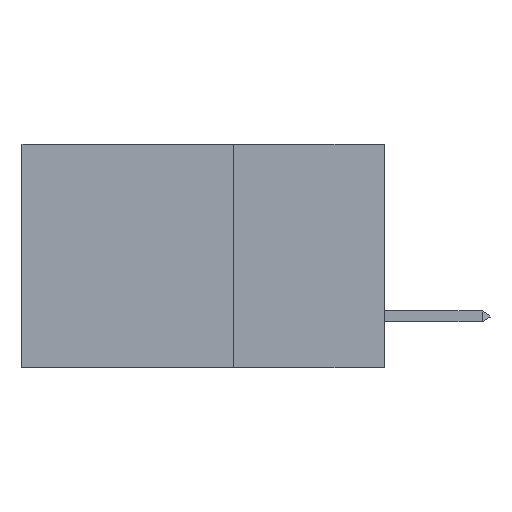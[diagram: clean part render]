
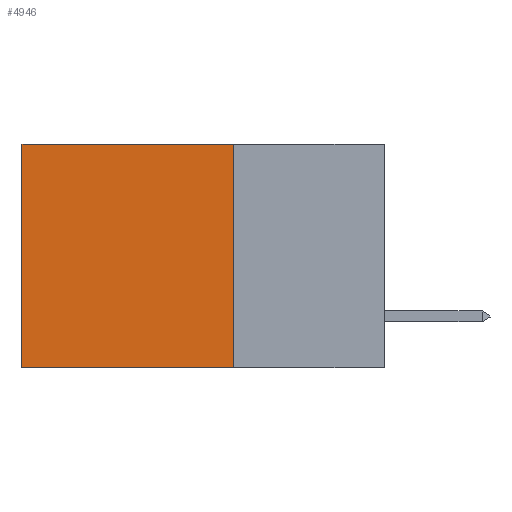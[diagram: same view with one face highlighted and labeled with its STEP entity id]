
A CAD part, left-side view. The second image highlights one B-rep face of the part: STEP entity #4946.
In plain terms, the highlighted planar face has unit normal (-1, 0, 0).
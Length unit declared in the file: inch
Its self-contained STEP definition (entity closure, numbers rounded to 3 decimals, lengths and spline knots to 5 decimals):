
#54 = VECTOR ( 'NONE', #7516, 39.37008 ) ;
#620 = VECTOR ( 'NONE', #25368, 39.37008 ) ;
#838 = EDGE_CURVE ( 'NONE', #45967, #17429, #23193, .T. ) ;
#1582 = CARTESIAN_POINT ( 'NONE',  ( 0.2875, 0.25, -0.37 ) ) ;
#3534 = LINE ( 'NONE', #39984, #35358 ) ;
#4235 = ORIENTED_EDGE ( 'NONE', *, *, #838, .T. ) ;
#4244 = ORIENTED_EDGE ( 'NONE', *, *, #40751, .F. ) ;
#4946 = ADVANCED_FACE ( 'NONE', ( #15515 ), #43310, .F. ) ;
#6645 = VERTEX_POINT ( 'NONE', #43587 ) ;
#7516 = DIRECTION ( 'NONE',  ( 0., 0., -1. ) ) ;
#9243 = LINE ( 'NONE', #11113, #54 ) ;
#11113 = CARTESIAN_POINT ( 'NONE',  ( 0.2875, 0.6, 0. ) ) ;
#12860 = AXIS2_PLACEMENT_3D ( 'NONE', #13928, #17624, #28800 ) ;
#12917 = EDGE_CURVE ( 'NONE', #17429, #42725, #9243, .T. ) ;
#13766 = DIRECTION ( 'NONE',  ( 0., 0., -1. ) ) ;
#13928 = CARTESIAN_POINT ( 'NONE',  ( 0.2875, 0.25, 0. ) ) ;
#14784 = CARTESIAN_POINT ( 'NONE',  ( 0.2875, 0.6, -0.37 ) ) ;
#15515 = FACE_OUTER_BOUND ( 'NONE', #17185, .T. ) ;
#17185 = EDGE_LOOP ( 'NONE', ( #27368, #4244, #46180, #4235 ) ) ;
#17429 = VERTEX_POINT ( 'NONE', #25997 ) ;
#17624 = DIRECTION ( 'NONE',  ( 1., 0., 0. ) ) ;
#23193 = LINE ( 'NONE', #43940, #620 ) ;
#25368 = DIRECTION ( 'NONE',  ( 0., 1., 0. ) ) ;
#25997 = CARTESIAN_POINT ( 'NONE',  ( 0.2875, 0.6, 0. ) ) ;
#26064 = EDGE_CURVE ( 'NONE', #45967, #6645, #3534, .T. ) ;
#27368 = ORIENTED_EDGE ( 'NONE', *, *, #12917, .T. ) ;
#28800 = DIRECTION ( 'NONE',  ( 0., 0., -1. ) ) ;
#32708 = CARTESIAN_POINT ( 'NONE',  ( 0.2875, 0.25, 0. ) ) ;
#35358 = VECTOR ( 'NONE', #13766, 39.37008 ) ;
#39984 = CARTESIAN_POINT ( 'NONE',  ( 0.2875, 0.25, 0. ) ) ;
#40751 = EDGE_CURVE ( 'NONE', #6645, #42725, #42546, .T. ) ;
#41366 = VECTOR ( 'NONE', #43876, 39.37008 ) ;
#42546 = LINE ( 'NONE', #1582, #41366 ) ;
#42725 = VERTEX_POINT ( 'NONE', #14784 ) ;
#43310 = PLANE ( 'NONE',  #12860 ) ;
#43587 = CARTESIAN_POINT ( 'NONE',  ( 0.2875, 0.25, -0.37 ) ) ;
#43876 = DIRECTION ( 'NONE',  ( 0., 1., 0. ) ) ;
#43940 = CARTESIAN_POINT ( 'NONE',  ( 0.2875, 0.25, 0. ) ) ;
#45967 = VERTEX_POINT ( 'NONE', #32708 ) ;
#46180 = ORIENTED_EDGE ( 'NONE', *, *, #26064, .F. ) ;
